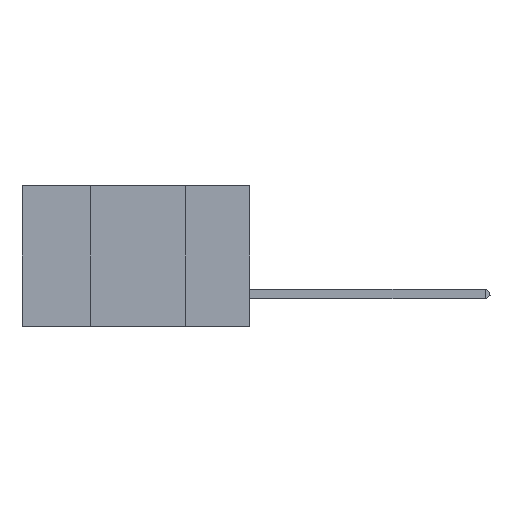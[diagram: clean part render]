
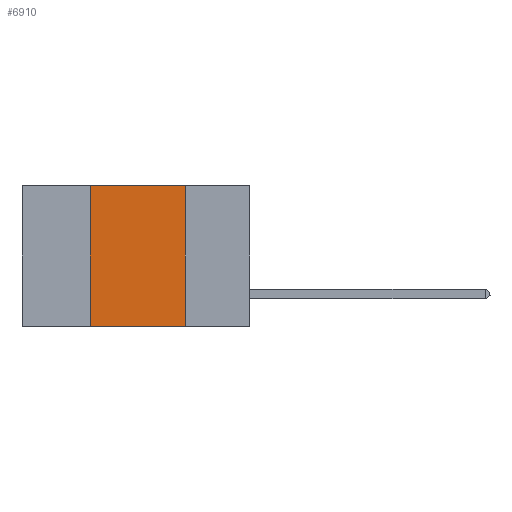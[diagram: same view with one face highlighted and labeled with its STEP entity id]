
A CAD part, left-side view. The second image highlights one B-rep face of the part: STEP entity #6910.
In plain terms, the highlighted planar face has unit normal (-1, 0, 0).
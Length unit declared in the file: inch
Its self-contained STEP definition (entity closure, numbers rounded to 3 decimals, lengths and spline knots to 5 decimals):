
#504 = DIRECTION ( 'NONE',  ( 0., 0., -1. ) ) ;
#559 = CARTESIAN_POINT ( 'NONE',  ( 0., 0.17, 0. ) ) ;
#1043 = EDGE_CURVE ( 'NONE', #13822, #13036, #18850, .T. ) ;
#1408 = CARTESIAN_POINT ( 'NONE',  ( 0., 0.42, 0. ) ) ;
#2529 = VECTOR ( 'NONE', #6851, 39.37008 ) ;
#3365 = ORIENTED_EDGE ( 'NONE', *, *, #11898, .F. ) ;
#4846 = VERTEX_POINT ( 'NONE', #1408 ) ;
#5009 = VECTOR ( 'NONE', #5687, 39.37008 ) ;
#5687 = DIRECTION ( 'NONE',  ( 0., -1., 0. ) ) ;
#5805 = EDGE_CURVE ( 'NONE', #4846, #5995, #19910, .T. ) ;
#5995 = VERTEX_POINT ( 'NONE', #10271 ) ;
#6583 = EDGE_LOOP ( 'NONE', ( #3365, #17489, #17791, #13931 ) ) ;
#6851 = DIRECTION ( 'NONE',  ( 0., 0., -1. ) ) ;
#6910 = ADVANCED_FACE ( 'NONE', ( #11380 ), #20080, .F. ) ;
#7625 = VECTOR ( 'NONE', #11247, 39.37008 ) ;
#7815 = CARTESIAN_POINT ( 'NONE',  ( 0., 0.42, 0. ) ) ;
#10241 = DIRECTION ( 'NONE',  ( 1., 0., 0. ) ) ;
#10271 = CARTESIAN_POINT ( 'NONE',  ( 0., 0.17, 0. ) ) ;
#10799 = CARTESIAN_POINT ( 'NONE',  ( 0., 0.6, 0. ) ) ;
#11247 = DIRECTION ( 'NONE',  ( 0., 0., 1. ) ) ;
#11380 = FACE_OUTER_BOUND ( 'NONE', #6583, .T. ) ;
#11733 = EDGE_CURVE ( 'NONE', #13822, #4846, #19690, .T. ) ;
#11898 = EDGE_CURVE ( 'NONE', #5995, #13036, #15860, .T. ) ;
#12525 = CARTESIAN_POINT ( 'NONE',  ( 0., 0.17, -0.37 ) ) ;
#13008 = CARTESIAN_POINT ( 'NONE',  ( 0., 0.42, -0.37 ) ) ;
#13036 = VERTEX_POINT ( 'NONE', #12525 ) ;
#13822 = VERTEX_POINT ( 'NONE', #13008 ) ;
#13931 = ORIENTED_EDGE ( 'NONE', *, *, #1043, .T. ) ;
#14513 = VECTOR ( 'NONE', #16209, 39.37008 ) ;
#15415 = CARTESIAN_POINT ( 'NONE',  ( 0., 0.6, 0. ) ) ;
#15860 = LINE ( 'NONE', #559, #2529 ) ;
#16209 = DIRECTION ( 'NONE',  ( 0., -1., 0. ) ) ;
#17489 = ORIENTED_EDGE ( 'NONE', *, *, #5805, .F. ) ;
#17791 = ORIENTED_EDGE ( 'NONE', *, *, #11733, .F. ) ;
#18635 = AXIS2_PLACEMENT_3D ( 'NONE', #15415, #10241, #504 ) ;
#18850 = LINE ( 'NONE', #19378, #14513 ) ;
#19378 = CARTESIAN_POINT ( 'NONE',  ( 0., 0.6, -0.37 ) ) ;
#19690 = LINE ( 'NONE', #7815, #7625 ) ;
#19910 = LINE ( 'NONE', #10799, #5009 ) ;
#20080 = PLANE ( 'NONE',  #18635 ) ;
